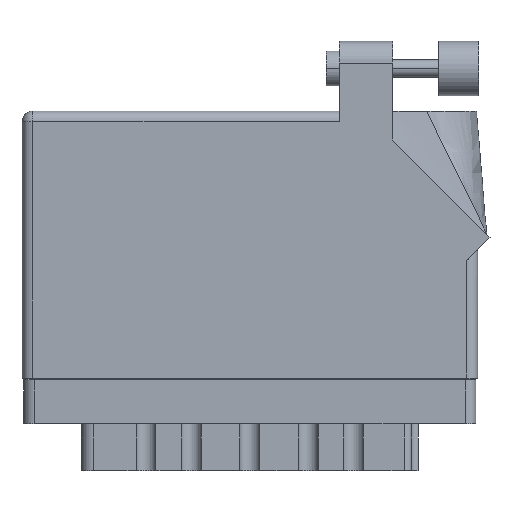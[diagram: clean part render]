
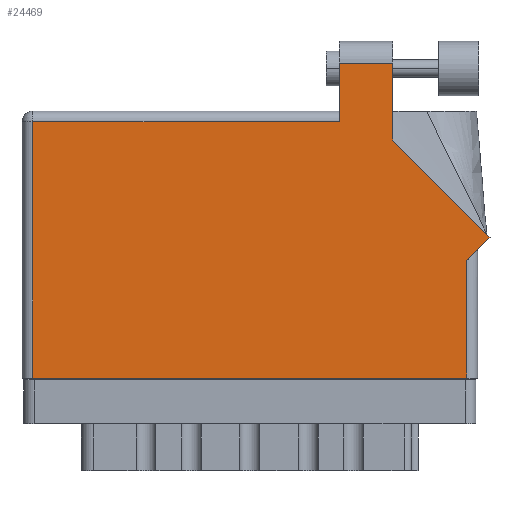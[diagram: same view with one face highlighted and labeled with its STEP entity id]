
A CAD part, front view. The second image highlights one B-rep face of the part: STEP entity #24469.
In plain terms, the highlighted face is planar.
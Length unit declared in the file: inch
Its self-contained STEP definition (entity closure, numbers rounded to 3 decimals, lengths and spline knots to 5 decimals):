
#853 = LINE ( 'NONE', #13846, #9108 ) ;
#1679 = LINE ( 'NONE', #47791, #35893 ) ;
#2617 = LINE ( 'NONE', #43855, #47410 ) ;
#3944 = ORIENTED_EDGE ( 'NONE', *, *, #46803, .T. ) ;
#5455 = EDGE_CURVE ( 'NONE', #8459, #33735, #17534, .T. ) ;
#6994 = VECTOR ( 'NONE', #21007, 39.37008 ) ;
#7161 = AXIS2_PLACEMENT_3D ( 'NONE', #40491, #36687, #11727 ) ;
#7363 = LINE ( 'NONE', #19859, #51066 ) ;
#8459 = VERTEX_POINT ( 'NONE', #50655 ) ;
#9108 = VECTOR ( 'NONE', #38527, 39.37008 ) ;
#9294 = VERTEX_POINT ( 'NONE', #23717 ) ;
#9805 = ORIENTED_EDGE ( 'NONE', *, *, #28614, .T. ) ;
#10831 = EDGE_LOOP ( 'NONE', ( #9805, #23622, #16775, #40660, #41509, #43647, #3944, #12233, #52207 ) ) ;
#11727 = DIRECTION ( 'NONE',  ( -1., 0., 0. ) ) ;
#12233 = ORIENTED_EDGE ( 'NONE', *, *, #28077, .T. ) ;
#12296 = LINE ( 'NONE', #28849, #6994 ) ;
#12439 = EDGE_CURVE ( 'NONE', #9294, #39330, #2617, .T. ) ;
#12514 = VECTOR ( 'NONE', #38751, 39.37008 ) ;
#13846 = CARTESIAN_POINT ( 'NONE',  ( 2.55, 0.737, 0. ) ) ;
#14377 = EDGE_CURVE ( 'NONE', #33735, #40194, #12296, .T. ) ;
#14715 = DIRECTION ( 'NONE',  ( 0., -1., 0. ) ) ;
#15471 = CARTESIAN_POINT ( 'NONE',  ( 1.819, 1.805, 0. ) ) ;
#16432 = CARTESIAN_POINT ( 'NONE',  ( 2.55, 0.675, 0. ) ) ;
#16775 = ORIENTED_EDGE ( 'NONE', *, *, #52829, .T. ) ;
#17534 = LINE ( 'NONE', #29741, #21578 ) ;
#18695 = LINE ( 'NONE', #22223, #12514 ) ;
#19038 = CARTESIAN_POINT ( 'NONE',  ( 2.68271, 0.80771, 0. ) ) ;
#19859 = CARTESIAN_POINT ( 'NONE',  ( 1.819, 1.53, 0. ) ) ;
#21007 = DIRECTION ( 'NONE',  ( 0., -1., 0. ) ) ;
#21578 = VECTOR ( 'NONE', #42192, 39.37008 ) ;
#22223 = CARTESIAN_POINT ( 'NONE',  ( 2.126, 1.36442, 0. ) ) ;
#23622 = ORIENTED_EDGE ( 'NONE', *, *, #12439, .T. ) ;
#23717 = CARTESIAN_POINT ( 'NONE',  ( 2.126, 1.805, 0. ) ) ;
#24469 = ADVANCED_FACE ( 'NONE', ( #40756 ), #24483, .F. ) ;
#24483 = PLANE ( 'NONE',  #7161 ) ;
#25016 = EDGE_CURVE ( 'NONE', #40194, #30851, #31785, .T. ) ;
#25077 = CARTESIAN_POINT ( 'NONE',  ( 0.062, 0., 0. ) ) ;
#25228 = VERTEX_POINT ( 'NONE', #49371 ) ;
#27723 = CARTESIAN_POINT ( 'NONE',  ( 0.062, 1.468, 0. ) ) ;
#28077 = EDGE_CURVE ( 'NONE', #50780, #28181, #1679, .T. ) ;
#28181 = VERTEX_POINT ( 'NONE', #19038 ) ;
#28614 = EDGE_CURVE ( 'NONE', #25228, #9294, #18695, .T. ) ;
#28849 = CARTESIAN_POINT ( 'NONE',  ( 0.062, 0., 0. ) ) ;
#29741 = CARTESIAN_POINT ( 'NONE',  ( 0., 1.468, 0. ) ) ;
#30851 = VERTEX_POINT ( 'NONE', #46786 ) ;
#31785 = LINE ( 'NONE', #48319, #43551 ) ;
#33571 = DIRECTION ( 'NONE',  ( -0.707, 0.707, 0. ) ) ;
#33735 = VERTEX_POINT ( 'NONE', #27723 ) ;
#33837 = LINE ( 'NONE', #46832, #53107 ) ;
#35893 = VECTOR ( 'NONE', #43162, 39.37008 ) ;
#36687 = DIRECTION ( 'NONE',  ( 0., 0., -1. ) ) ;
#38527 = DIRECTION ( 'NONE',  ( 0., 1., 0. ) ) ;
#38751 = DIRECTION ( 'NONE',  ( 0., 1., 0. ) ) ;
#39330 = VERTEX_POINT ( 'NONE', #15471 ) ;
#40194 = VERTEX_POINT ( 'NONE', #25077 ) ;
#40491 = CARTESIAN_POINT ( 'NONE',  ( 0., 1.53, 0. ) ) ;
#40660 = ORIENTED_EDGE ( 'NONE', *, *, #5455, .T. ) ;
#40756 = FACE_OUTER_BOUND ( 'NONE', #10831, .T. ) ;
#40842 = DIRECTION ( 'NONE',  ( -1., 0., 0. ) ) ;
#41094 = EDGE_CURVE ( 'NONE', #28181, #25228, #33837, .T. ) ;
#41509 = ORIENTED_EDGE ( 'NONE', *, *, #14377, .T. ) ;
#42192 = DIRECTION ( 'NONE',  ( -1., 0., 0. ) ) ;
#43162 = DIRECTION ( 'NONE',  ( 0.707, 0.707, 0. ) ) ;
#43551 = VECTOR ( 'NONE', #44507, 39.37008 ) ;
#43647 = ORIENTED_EDGE ( 'NONE', *, *, #25016, .T. ) ;
#43855 = CARTESIAN_POINT ( 'NONE',  ( 1.819, 1.805, 0. ) ) ;
#44507 = DIRECTION ( 'NONE',  ( 1., 0., 0. ) ) ;
#46786 = CARTESIAN_POINT ( 'NONE',  ( 2.55, 0., 0. ) ) ;
#46803 = EDGE_CURVE ( 'NONE', #30851, #50780, #853, .T. ) ;
#46832 = CARTESIAN_POINT ( 'NONE',  ( 2.68271, 0.80771, 0. ) ) ;
#47410 = VECTOR ( 'NONE', #40842, 39.37008 ) ;
#47791 = CARTESIAN_POINT ( 'NONE',  ( 2.612, 0.737, 0. ) ) ;
#48319 = CARTESIAN_POINT ( 'NONE',  ( 0., 0., 0. ) ) ;
#49371 = CARTESIAN_POINT ( 'NONE',  ( 2.126, 1.36442, 0. ) ) ;
#50655 = CARTESIAN_POINT ( 'NONE',  ( 1.819, 1.468, 0. ) ) ;
#50780 = VERTEX_POINT ( 'NONE', #16432 ) ;
#51066 = VECTOR ( 'NONE', #14715, 39.37008 ) ;
#52207 = ORIENTED_EDGE ( 'NONE', *, *, #41094, .T. ) ;
#52829 = EDGE_CURVE ( 'NONE', #39330, #8459, #7363, .T. ) ;
#53107 = VECTOR ( 'NONE', #33571, 39.37008 ) ;
